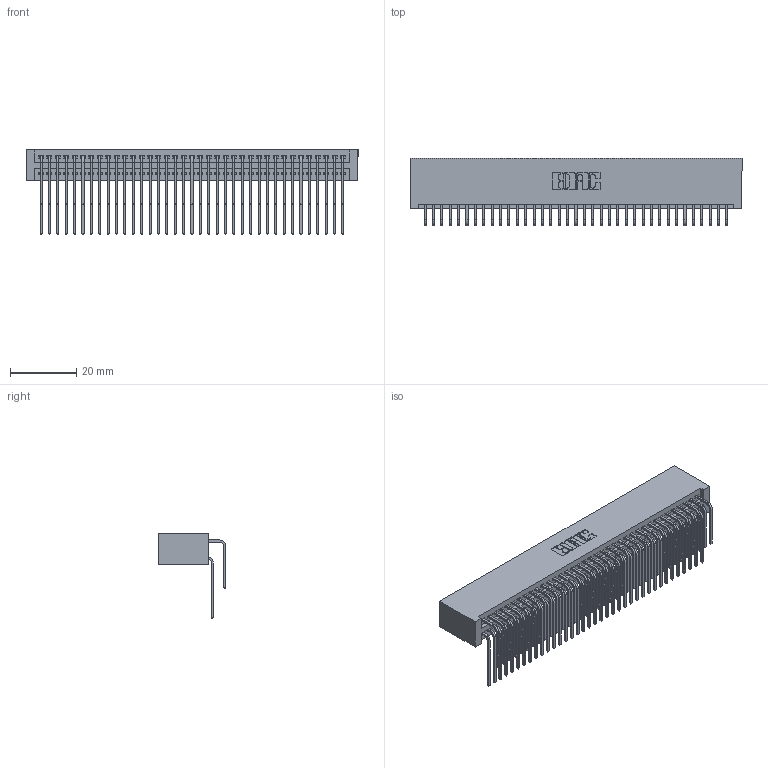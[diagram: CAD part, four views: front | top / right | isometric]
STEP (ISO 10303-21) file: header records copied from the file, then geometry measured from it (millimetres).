
FILE_DESCRIPTION (( 'STEP AP203' ), '1' );
FILE_NAME ('345-074-559-201.STEP', '2018-10-02T14:03:30', ( '' ), ( '' ), 'SwSTEP 2.0', 'SolidWorks 2016', '' );
FILE_SCHEMA (( 'CONFIG_CONTROL_DESIGN' ));
Length unit declared in the file: inch
Products named in the file (4): 345 Part_No Mounting Lugs; 345-292-001_558 559 Tail - 1; 345-292-001_559 Tail - 2; 345-074-559-201
Assembly tree (75 placements, depth 2):
  345-074-559-201
    345 Part_No Mounting Lugs
    345-292-001_558 559 Tail - 1  x37
    345-292-001_559 Tail - 2  x37
Bounding box: 100.58 x 20.56 x 25.53 mm (x, y, z)
Volume: 10767.2 mm3; surface area: 18129.5 mm2
Topology: 75 solids, 75 shells, 3966 faces, 11787 edges, 7758 vertices
Faces by surface type: plane 2666, cylinder 1300
Entity records: 31079 total; most frequent: CARTESIAN_POINT 5259, ORIENTED_EDGE 5142, DIRECTION 4611, EDGE_CURVE 2571, VECTOR 2259, LINE 2259, VERTEX_POINT 1710, AXIS2_PLACEMENT_3D 1176
